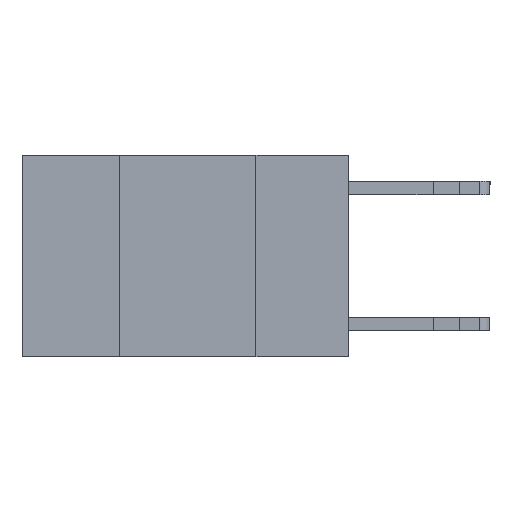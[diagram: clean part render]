
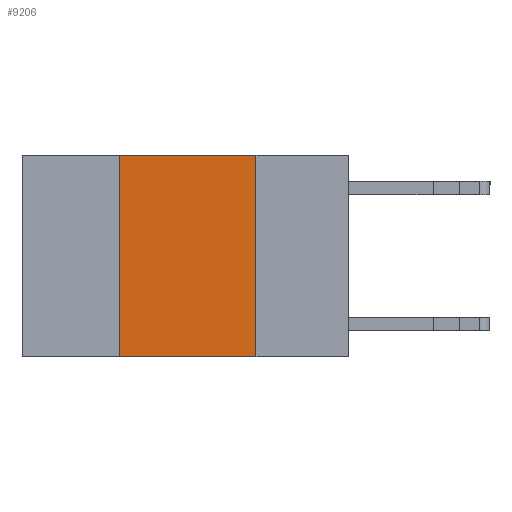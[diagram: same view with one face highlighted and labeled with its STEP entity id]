
A CAD part, left-side view. The second image highlights one B-rep face of the part: STEP entity #9206.
In plain terms, the highlighted planar face has unit normal (-1, 0, 0).
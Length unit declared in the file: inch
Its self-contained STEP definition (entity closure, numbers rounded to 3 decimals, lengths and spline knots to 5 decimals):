
#243 = CARTESIAN_POINT ( 'NONE',  ( 0., 0.17, -0.37 ) ) ;
#372 = AXIS2_PLACEMENT_3D ( 'NONE', #18567, #12463, #14287 ) ;
#703 = VECTOR ( 'NONE', #13076, 39.37008 ) ;
#1169 = CARTESIAN_POINT ( 'NONE',  ( 0., 0.6, 0. ) ) ;
#1923 = CARTESIAN_POINT ( 'NONE',  ( 0., 0.42, 0. ) ) ;
#2397 = EDGE_LOOP ( 'NONE', ( #15840, #11811, #13575, #3887 ) ) ;
#2495 = LINE ( 'NONE', #12042, #4923 ) ;
#2558 = EDGE_CURVE ( 'NONE', #10883, #2890, #2495, .T. ) ;
#2890 = VERTEX_POINT ( 'NONE', #243 ) ;
#3250 = DIRECTION ( 'NONE',  ( 0., 0., 1. ) ) ;
#3281 = EDGE_CURVE ( 'NONE', #9083, #2890, #14932, .T. ) ;
#3364 = DIRECTION ( 'NONE',  ( 0., -1., 0. ) ) ;
#3887 = ORIENTED_EDGE ( 'NONE', *, *, #2558, .T. ) ;
#4923 = VECTOR ( 'NONE', #3364, 39.37008 ) ;
#5674 = VERTEX_POINT ( 'NONE', #1923 ) ;
#5893 = EDGE_CURVE ( 'NONE', #10883, #5674, #12225, .T. ) ;
#7001 = PLANE ( 'NONE',  #372 ) ;
#7231 = CARTESIAN_POINT ( 'NONE',  ( 0., 0.42, 0. ) ) ;
#7573 = CARTESIAN_POINT ( 'NONE',  ( 0., 0.17, 0. ) ) ;
#9083 = VERTEX_POINT ( 'NONE', #7573 ) ;
#9206 = ADVANCED_FACE ( 'NONE', ( #18659 ), #7001, .F. ) ;
#10417 = CARTESIAN_POINT ( 'NONE',  ( 0., 0.42, -0.37 ) ) ;
#10883 = VERTEX_POINT ( 'NONE', #10417 ) ;
#11811 = ORIENTED_EDGE ( 'NONE', *, *, #18144, .F. ) ;
#12042 = CARTESIAN_POINT ( 'NONE',  ( 0., 0.6, -0.37 ) ) ;
#12173 = DIRECTION ( 'NONE',  ( 0., 0., -1. ) ) ;
#12225 = LINE ( 'NONE', #7231, #12826 ) ;
#12463 = DIRECTION ( 'NONE',  ( 1., 0., 0. ) ) ;
#12826 = VECTOR ( 'NONE', #3250, 39.37008 ) ;
#13076 = DIRECTION ( 'NONE',  ( 0., -1., 0. ) ) ;
#13575 = ORIENTED_EDGE ( 'NONE', *, *, #5893, .F. ) ;
#14287 = DIRECTION ( 'NONE',  ( 0., 0., -1. ) ) ;
#14696 = VECTOR ( 'NONE', #12173, 39.37008 ) ;
#14932 = LINE ( 'NONE', #15229, #14696 ) ;
#15229 = CARTESIAN_POINT ( 'NONE',  ( 0., 0.17, 0. ) ) ;
#15840 = ORIENTED_EDGE ( 'NONE', *, *, #3281, .F. ) ;
#18144 = EDGE_CURVE ( 'NONE', #5674, #9083, #18540, .T. ) ;
#18540 = LINE ( 'NONE', #1169, #703 ) ;
#18567 = CARTESIAN_POINT ( 'NONE',  ( 0., 0.6, 0. ) ) ;
#18659 = FACE_OUTER_BOUND ( 'NONE', #2397, .T. ) ;
